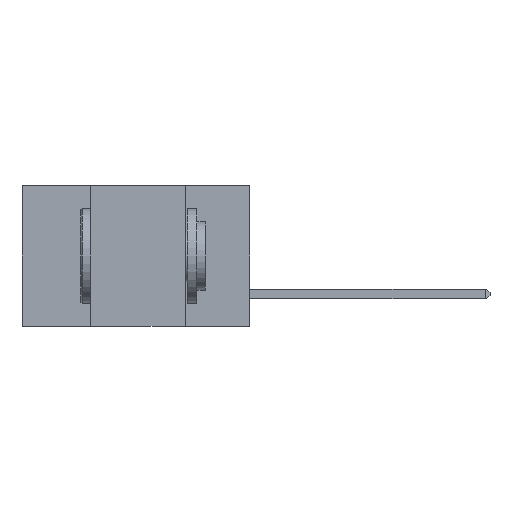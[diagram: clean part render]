
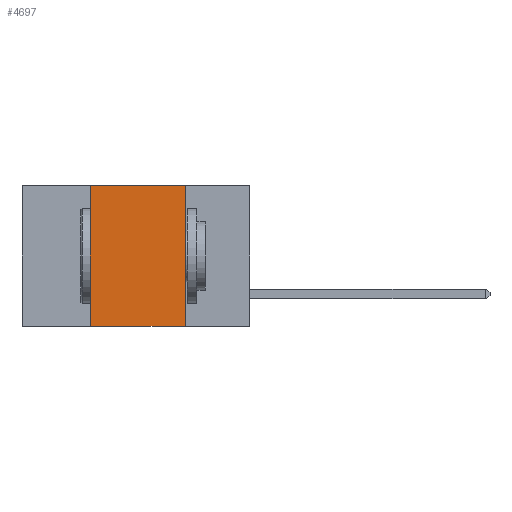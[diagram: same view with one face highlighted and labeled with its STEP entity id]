
A CAD part, left-side view. The second image highlights one B-rep face of the part: STEP entity #4697.
In plain terms, the highlighted planar face has unit normal (-1, 0, 0).
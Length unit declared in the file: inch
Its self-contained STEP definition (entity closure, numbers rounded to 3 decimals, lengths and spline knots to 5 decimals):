
#26 = FACE_OUTER_BOUND ( 'NONE', #8502, .T. ) ;
#308 = CARTESIAN_POINT ( 'NONE',  ( 0., 0.17, 0. ) ) ;
#792 = VECTOR ( 'NONE', #11044, 39.37008 ) ;
#1236 = ORIENTED_EDGE ( 'NONE', *, *, #8874, .F. ) ;
#3062 = CARTESIAN_POINT ( 'NONE',  ( 0., 0.42, 0. ) ) ;
#3102 = VERTEX_POINT ( 'NONE', #3062 ) ;
#3197 = CARTESIAN_POINT ( 'NONE',  ( 0., 0.42, -0.37 ) ) ;
#3374 = LINE ( 'NONE', #11143, #792 ) ;
#3425 = VERTEX_POINT ( 'NONE', #308 ) ;
#3474 = ORIENTED_EDGE ( 'NONE', *, *, #8713, .F. ) ;
#3573 = DIRECTION ( 'NONE',  ( 0., 0., 1. ) ) ;
#3784 = ORIENTED_EDGE ( 'NONE', *, *, #9098, .T. ) ;
#4163 = VECTOR ( 'NONE', #12009, 39.37008 ) ;
#4697 = ADVANCED_FACE ( 'NONE', ( #26 ), #5076, .F. ) ;
#5015 = DIRECTION ( 'NONE',  ( 0., 0., -1. ) ) ;
#5043 = DIRECTION ( 'NONE',  ( 1., 0., 0. ) ) ;
#5076 = PLANE ( 'NONE',  #6087 ) ;
#5110 = CARTESIAN_POINT ( 'NONE',  ( 0., 0.6, 0. ) ) ;
#5276 = EDGE_CURVE ( 'NONE', #3102, #3425, #3374, .T. ) ;
#5390 = VERTEX_POINT ( 'NONE', #10069 ) ;
#6087 = AXIS2_PLACEMENT_3D ( 'NONE', #5110, #5043, #5015 ) ;
#6734 = LINE ( 'NONE', #11194, #4163 ) ;
#6898 = VECTOR ( 'NONE', #3573, 39.37008 ) ;
#8328 = CARTESIAN_POINT ( 'NONE',  ( 0., 0.42, 0. ) ) ;
#8363 = LINE ( 'NONE', #10814, #10722 ) ;
#8502 = EDGE_LOOP ( 'NONE', ( #3474, #8552, #1236, #3784 ) ) ;
#8530 = VERTEX_POINT ( 'NONE', #3197 ) ;
#8552 = ORIENTED_EDGE ( 'NONE', *, *, #5276, .F. ) ;
#8713 = EDGE_CURVE ( 'NONE', #3425, #5390, #8363, .T. ) ;
#8874 = EDGE_CURVE ( 'NONE', #8530, #3102, #9067, .T. ) ;
#9067 = LINE ( 'NONE', #8328, #6898 ) ;
#9098 = EDGE_CURVE ( 'NONE', #8530, #5390, #6734, .T. ) ;
#10069 = CARTESIAN_POINT ( 'NONE',  ( 0., 0.17, -0.37 ) ) ;
#10722 = VECTOR ( 'NONE', #11624, 39.37008 ) ;
#10814 = CARTESIAN_POINT ( 'NONE',  ( 0., 0.17, 0. ) ) ;
#11044 = DIRECTION ( 'NONE',  ( 0., -1., 0. ) ) ;
#11143 = CARTESIAN_POINT ( 'NONE',  ( 0., 0.6, 0. ) ) ;
#11194 = CARTESIAN_POINT ( 'NONE',  ( 0., 0.6, -0.37 ) ) ;
#11624 = DIRECTION ( 'NONE',  ( 0., 0., -1. ) ) ;
#12009 = DIRECTION ( 'NONE',  ( 0., -1., 0. ) ) ;
